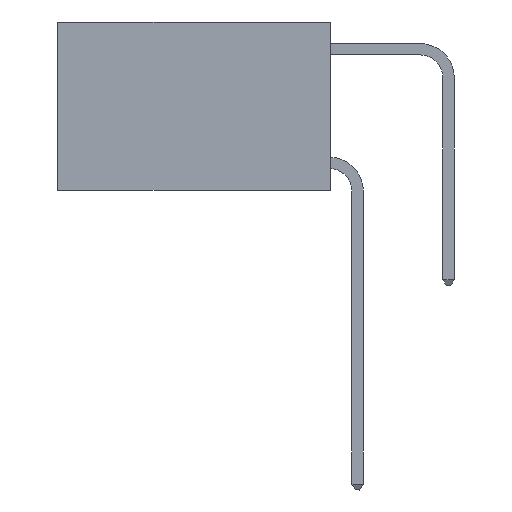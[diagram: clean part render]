
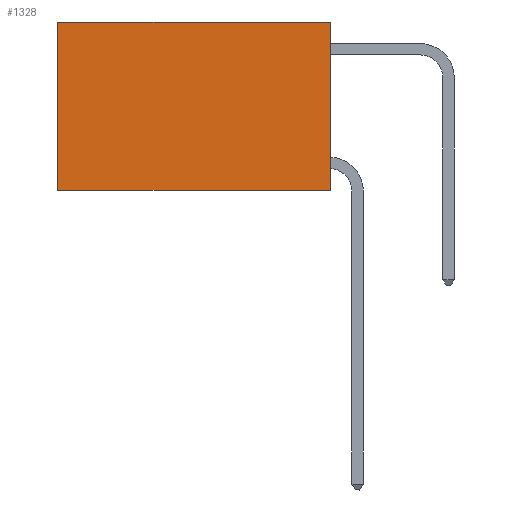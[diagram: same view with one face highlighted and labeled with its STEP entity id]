
A CAD part, left-side view. The second image highlights one B-rep face of the part: STEP entity #1328.
In plain terms, the highlighted planar face has unit normal (-1, 0, 0).
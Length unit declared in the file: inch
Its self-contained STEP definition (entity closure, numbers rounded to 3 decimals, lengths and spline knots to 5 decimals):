
#219 = DIRECTION ( 'NONE',  ( 0., 1., 0. ) ) ;
#441 = LINE ( 'NONE', #12005, #23900 ) ;
#1328 = ADVANCED_FACE ( 'NONE', ( #23832 ), #22154, .F. ) ;
#1786 = ORIENTED_EDGE ( 'NONE', *, *, #8761, .F. ) ;
#1935 = CARTESIAN_POINT ( 'NONE',  ( 0.2625, 0., -0.37 ) ) ;
#2406 = CARTESIAN_POINT ( 'NONE',  ( 0.2625, 0., 0. ) ) ;
#4041 = ORIENTED_EDGE ( 'NONE', *, *, #21370, .T. ) ;
#4975 = ORIENTED_EDGE ( 'NONE', *, *, #16017, .F. ) ;
#6120 = LINE ( 'NONE', #11892, #19455 ) ;
#6196 = ORIENTED_EDGE ( 'NONE', *, *, #13093, .T. ) ;
#6445 = CARTESIAN_POINT ( 'NONE',  ( 0.2625, 0., 0. ) ) ;
#6698 = LINE ( 'NONE', #6445, #12834 ) ;
#6878 = VECTOR ( 'NONE', #19269, 39.37008 ) ;
#8761 = EDGE_CURVE ( 'NONE', #10554, #23484, #6698, .T. ) ;
#10244 = DIRECTION ( 'NONE',  ( 0., 0., -1. ) ) ;
#10554 = VERTEX_POINT ( 'NONE', #14502 ) ;
#10753 = DIRECTION ( 'NONE',  ( 1., 0., 0. ) ) ;
#11892 = CARTESIAN_POINT ( 'NONE',  ( 0.2625, 0., 0. ) ) ;
#12005 = CARTESIAN_POINT ( 'NONE',  ( 0.2625, 0.6, 0. ) ) ;
#12351 = DIRECTION ( 'NONE',  ( 0., 0., -1. ) ) ;
#12834 = VECTOR ( 'NONE', #12351, 39.37008 ) ;
#13093 = EDGE_CURVE ( 'NONE', #10554, #20896, #6120, .T. ) ;
#13524 = CARTESIAN_POINT ( 'NONE',  ( 0.2625, 0., -0.37 ) ) ;
#14502 = CARTESIAN_POINT ( 'NONE',  ( 0.2625, 0., 0. ) ) ;
#16017 = EDGE_CURVE ( 'NONE', #23484, #20765, #23774, .T. ) ;
#17930 = EDGE_LOOP ( 'NONE', ( #4041, #4975, #1786, #6196 ) ) ;
#19269 = DIRECTION ( 'NONE',  ( 0., 1., 0. ) ) ;
#19455 = VECTOR ( 'NONE', #219, 39.37008 ) ;
#19716 = CARTESIAN_POINT ( 'NONE',  ( 0.2625, 0.6, 0. ) ) ;
#19803 = DIRECTION ( 'NONE',  ( 0., 0., -1. ) ) ;
#20765 = VERTEX_POINT ( 'NONE', #20901 ) ;
#20896 = VERTEX_POINT ( 'NONE', #19716 ) ;
#20901 = CARTESIAN_POINT ( 'NONE',  ( 0.2625, 0.6, -0.37 ) ) ;
#21370 = EDGE_CURVE ( 'NONE', #20896, #20765, #441, .T. ) ;
#22154 = PLANE ( 'NONE',  #25267 ) ;
#23484 = VERTEX_POINT ( 'NONE', #1935 ) ;
#23774 = LINE ( 'NONE', #13524, #6878 ) ;
#23832 = FACE_OUTER_BOUND ( 'NONE', #17930, .T. ) ;
#23900 = VECTOR ( 'NONE', #19803, 39.37008 ) ;
#25267 = AXIS2_PLACEMENT_3D ( 'NONE', #2406, #10753, #10244 ) ;
